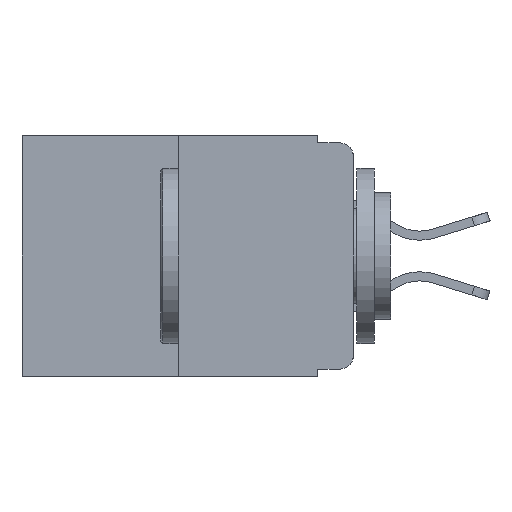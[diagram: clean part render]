
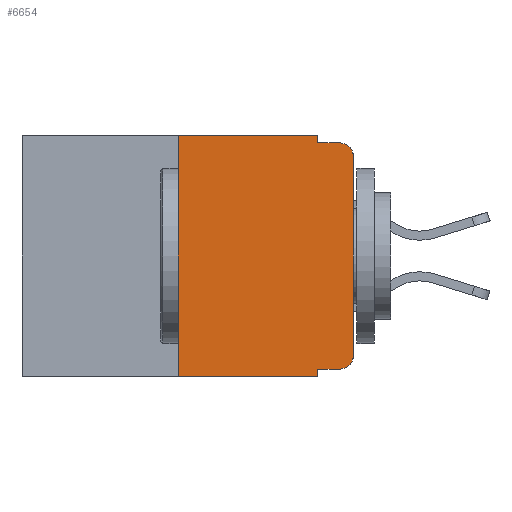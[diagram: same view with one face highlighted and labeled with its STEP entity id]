
A CAD part, left-side view. The second image highlights one B-rep face of the part: STEP entity #6654.
In plain terms, the highlighted planar face has unit normal (-1, 0, 0).
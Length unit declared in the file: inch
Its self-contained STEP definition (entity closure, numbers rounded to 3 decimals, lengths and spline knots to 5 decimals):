
#120 = EDGE_CURVE ( 'NONE', #6138, #827, #13166, .T. ) ;
#261 = LINE ( 'NONE', #8435, #8900 ) ;
#554 = ORIENTED_EDGE ( 'NONE', *, *, #1486, .F. ) ;
#617 = DIRECTION ( 'NONE',  ( 0., 0., -1. ) ) ;
#827 = VERTEX_POINT ( 'NONE', #11655 ) ;
#943 = EDGE_CURVE ( 'NONE', #5722, #8065, #3028, .T. ) ;
#1315 = VERTEX_POINT ( 'NONE', #11628 ) ;
#1368 = ORIENTED_EDGE ( 'NONE', *, *, #1596, .T. ) ;
#1431 = EDGE_CURVE ( 'NONE', #2484, #10064, #1930, .T. ) ;
#1437 = EDGE_CURVE ( 'NONE', #10064, #1315, #5456, .T. ) ;
#1476 = EDGE_CURVE ( 'NONE', #13392, #1315, #9606, .T. ) ;
#1483 = EDGE_CURVE ( 'NONE', #827, #13392, #261, .T. ) ;
#1486 = EDGE_CURVE ( 'NONE', #5722, #6138, #3332, .T. ) ;
#1534 = EDGE_CURVE ( 'NONE', #9537, #8065, #4581, .T. ) ;
#1542 = EDGE_CURVE ( 'NONE', #9537, #9021, #10092, .T. ) ;
#1596 = EDGE_CURVE ( 'NONE', #9021, #2484, #3532, .T. ) ;
#1818 = DIRECTION ( 'NONE',  ( 0., 0., 1. ) ) ;
#1930 = LINE ( 'NONE', #8466, #10580 ) ;
#2230 = CARTESIAN_POINT ( 'NONE',  ( 0., 0.473, 0. ) ) ;
#2484 = VERTEX_POINT ( 'NONE', #3164 ) ;
#2591 = DIRECTION ( 'NONE',  ( 0., 0., -1. ) ) ;
#2621 = DIRECTION ( 'NONE',  ( -1., 0., 0. ) ) ;
#2688 = AXIS2_PLACEMENT_3D ( 'NONE', #12558, #12542, #617 ) ;
#2824 = ORIENTED_EDGE ( 'NONE', *, *, #1437, .T. ) ;
#3028 = LINE ( 'NONE', #12396, #8615 ) ;
#3164 = CARTESIAN_POINT ( 'NONE',  ( 0., 0., -0.313 ) ) ;
#3332 = LINE ( 'NONE', #10494, #13945 ) ;
#3532 = CIRCLE ( 'NONE', #14147, 0.02 ) ;
#3556 = PLANE ( 'NONE',  #10652 ) ;
#3579 = CARTESIAN_POINT ( 'NONE',  ( 0., 0.051, -0.333 ) ) ;
#3849 = CARTESIAN_POINT ( 'NONE',  ( 0., 0.051, -0.01 ) ) ;
#3961 = ORIENTED_EDGE ( 'NONE', *, *, #943, .T. ) ;
#4243 = VECTOR ( 'NONE', #13909, 39.37008 ) ;
#4321 = ORIENTED_EDGE ( 'NONE', *, *, #1542, .T. ) ;
#4581 = LINE ( 'NONE', #7939, #12756 ) ;
#4689 = DIRECTION ( 'NONE',  ( 1., 0., 0. ) ) ;
#5249 = CARTESIAN_POINT ( 'NONE',  ( 0., 0.051, -0.01 ) ) ;
#5456 = CIRCLE ( 'NONE', #2688, 0.02 ) ;
#5634 = DIRECTION ( 'NONE',  ( 0., 0., -1. ) ) ;
#5664 = CARTESIAN_POINT ( 'NONE',  ( 0., 0.25, -0.343 ) ) ;
#5722 = VERTEX_POINT ( 'NONE', #5664 ) ;
#5861 = ORIENTED_EDGE ( 'NONE', *, *, #1476, .F. ) ;
#5880 = DIRECTION ( 'NONE',  ( 0., 0., 1. ) ) ;
#6138 = VERTEX_POINT ( 'NONE', #11597 ) ;
#6187 = ORIENTED_EDGE ( 'NONE', *, *, #120, .F. ) ;
#6208 = CARTESIAN_POINT ( 'NONE',  ( 0., 0.051, -0.343 ) ) ;
#6285 = VECTOR ( 'NONE', #12294, 39.37008 ) ;
#6654 = ADVANCED_FACE ( 'NONE', ( #11246 ), #3556, .F. ) ;
#7601 = VECTOR ( 'NONE', #9379, 39.37008 ) ;
#7611 = CARTESIAN_POINT ( 'NONE',  ( 0., 0.473, 0. ) ) ;
#7939 = CARTESIAN_POINT ( 'NONE',  ( 0., 0.051, 0. ) ) ;
#8065 = VERTEX_POINT ( 'NONE', #6208 ) ;
#8249 = CARTESIAN_POINT ( 'NONE',  ( 0., 0.02, -0.333 ) ) ;
#8427 = ORIENTED_EDGE ( 'NONE', *, *, #1431, .T. ) ;
#8435 = CARTESIAN_POINT ( 'NONE',  ( 0., 0.051, 0. ) ) ;
#8466 = CARTESIAN_POINT ( 'NONE',  ( 0., 0., 0. ) ) ;
#8615 = VECTOR ( 'NONE', #10701, 39.37008 ) ;
#8637 = CARTESIAN_POINT ( 'NONE',  ( 0., 0., -0.03 ) ) ;
#8790 = ORIENTED_EDGE ( 'NONE', *, *, #1483, .F. ) ;
#8900 = VECTOR ( 'NONE', #12865, 39.37008 ) ;
#9021 = VERTEX_POINT ( 'NONE', #8249 ) ;
#9379 = DIRECTION ( 'NONE',  ( 0., -1., 0. ) ) ;
#9537 = VERTEX_POINT ( 'NONE', #3579 ) ;
#9606 = LINE ( 'NONE', #5249, #6285 ) ;
#9844 = ORIENTED_EDGE ( 'NONE', *, *, #1534, .F. ) ;
#10064 = VERTEX_POINT ( 'NONE', #8637 ) ;
#10092 = LINE ( 'NONE', #13281, #4243 ) ;
#10494 = CARTESIAN_POINT ( 'NONE',  ( 0., 0.25, 0. ) ) ;
#10580 = VECTOR ( 'NONE', #5880, 39.37008 ) ;
#10652 = AXIS2_PLACEMENT_3D ( 'NONE', #2230, #4689, #12200 ) ;
#10701 = DIRECTION ( 'NONE',  ( 0., -1., 0. ) ) ;
#11246 = FACE_OUTER_BOUND ( 'NONE', #12045, .T. ) ;
#11597 = CARTESIAN_POINT ( 'NONE',  ( 0., 0.25, 0. ) ) ;
#11628 = CARTESIAN_POINT ( 'NONE',  ( 0., 0.02, -0.01 ) ) ;
#11655 = CARTESIAN_POINT ( 'NONE',  ( 0., 0.051, 0. ) ) ;
#12045 = EDGE_LOOP ( 'NONE', ( #8427, #2824, #5861, #8790, #6187, #554, #3961, #9844, #4321, #1368 ) ) ;
#12200 = DIRECTION ( 'NONE',  ( 0., 0., -1. ) ) ;
#12294 = DIRECTION ( 'NONE',  ( 0., -1., 0. ) ) ;
#12396 = CARTESIAN_POINT ( 'NONE',  ( 0., 0.473, -0.343 ) ) ;
#12542 = DIRECTION ( 'NONE',  ( -1., 0., 0. ) ) ;
#12558 = CARTESIAN_POINT ( 'NONE',  ( 0., 0.02, -0.03 ) ) ;
#12756 = VECTOR ( 'NONE', #5634, 39.37008 ) ;
#12865 = DIRECTION ( 'NONE',  ( 0., 0., -1. ) ) ;
#12938 = CARTESIAN_POINT ( 'NONE',  ( 0., 0.02, -0.313 ) ) ;
#13166 = LINE ( 'NONE', #7611, #7601 ) ;
#13281 = CARTESIAN_POINT ( 'NONE',  ( 0., 0.051, -0.333 ) ) ;
#13392 = VERTEX_POINT ( 'NONE', #3849 ) ;
#13909 = DIRECTION ( 'NONE',  ( 0., -1., 0. ) ) ;
#13945 = VECTOR ( 'NONE', #1818, 39.37008 ) ;
#14147 = AXIS2_PLACEMENT_3D ( 'NONE', #12938, #2621, #2591 ) ;
